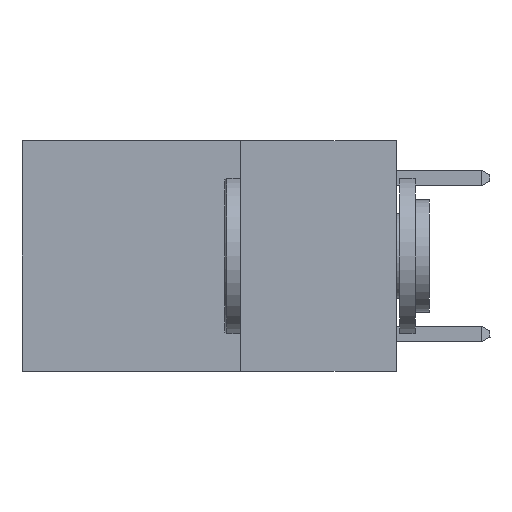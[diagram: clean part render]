
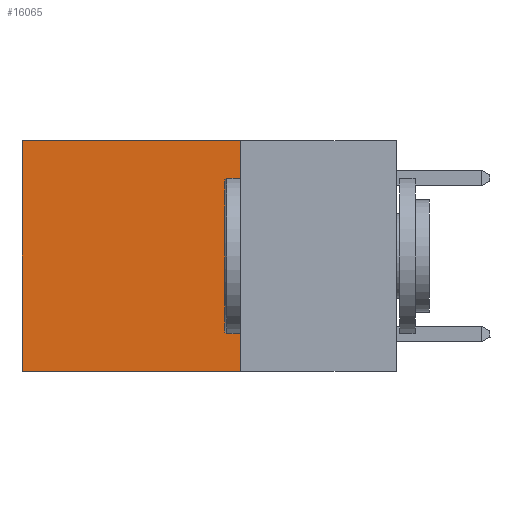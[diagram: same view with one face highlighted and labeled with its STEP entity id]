
A CAD part, left-side view. The second image highlights one B-rep face of the part: STEP entity #16065.
In plain terms, the highlighted planar face has unit normal (-1, 0, 0).
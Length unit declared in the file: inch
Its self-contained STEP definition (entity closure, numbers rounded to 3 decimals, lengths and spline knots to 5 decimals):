
#201 = VERTEX_POINT ( 'NONE', #2603 ) ;
#833 = VECTOR ( 'NONE', #1078, 39.37008 ) ;
#1078 = DIRECTION ( 'NONE',  ( 0., 1., 0. ) ) ;
#1350 = DIRECTION ( 'NONE',  ( 0., 0., -1. ) ) ;
#2198 = CARTESIAN_POINT ( 'NONE',  ( 0.2625, 0.25, 0. ) ) ;
#2397 = LINE ( 'NONE', #16668, #16218 ) ;
#2441 = FACE_OUTER_BOUND ( 'NONE', #7297, .T. ) ;
#2603 = CARTESIAN_POINT ( 'NONE',  ( 0.2625, 0.6, 0. ) ) ;
#3335 = ORIENTED_EDGE ( 'NONE', *, *, #18366, .T. ) ;
#4083 = EDGE_CURVE ( 'NONE', #201, #9149, #12155, .T. ) ;
#5642 = CARTESIAN_POINT ( 'NONE',  ( 0.2625, 0.25, 0. ) ) ;
#6493 = VECTOR ( 'NONE', #1350, 39.37008 ) ;
#7297 = EDGE_LOOP ( 'NONE', ( #19513, #7813, #15639, #3335 ) ) ;
#7525 = CARTESIAN_POINT ( 'NONE',  ( 0.2625, 0.25, -0.37 ) ) ;
#7813 = ORIENTED_EDGE ( 'NONE', *, *, #8856, .F. ) ;
#8118 = VERTEX_POINT ( 'NONE', #7525 ) ;
#8508 = DIRECTION ( 'NONE',  ( 1., 0., 0. ) ) ;
#8566 = DIRECTION ( 'NONE',  ( 0., 0., -1. ) ) ;
#8856 = EDGE_CURVE ( 'NONE', #8118, #9149, #19380, .T. ) ;
#9149 = VERTEX_POINT ( 'NONE', #13973 ) ;
#10589 = DIRECTION ( 'NONE',  ( 0., 0., -1. ) ) ;
#11029 = VERTEX_POINT ( 'NONE', #5642 ) ;
#11312 = CARTESIAN_POINT ( 'NONE',  ( 0.2625, 0.25, -0.37 ) ) ;
#12155 = LINE ( 'NONE', #16631, #6493 ) ;
#13565 = CARTESIAN_POINT ( 'NONE',  ( 0.2625, 0.25, 0. ) ) ;
#13973 = CARTESIAN_POINT ( 'NONE',  ( 0.2625, 0.6, -0.37 ) ) ;
#14780 = PLANE ( 'NONE',  #16892 ) ;
#15639 = ORIENTED_EDGE ( 'NONE', *, *, #18298, .F. ) ;
#15897 = DIRECTION ( 'NONE',  ( 0., 1., 0. ) ) ;
#16065 = ADVANCED_FACE ( 'NONE', ( #2441 ), #14780, .F. ) ;
#16218 = VECTOR ( 'NONE', #8566, 39.37008 ) ;
#16631 = CARTESIAN_POINT ( 'NONE',  ( 0.2625, 0.6, 0. ) ) ;
#16668 = CARTESIAN_POINT ( 'NONE',  ( 0.2625, 0.25, 0. ) ) ;
#16892 = AXIS2_PLACEMENT_3D ( 'NONE', #13565, #8508, #10589 ) ;
#18002 = LINE ( 'NONE', #2198, #833 ) ;
#18298 = EDGE_CURVE ( 'NONE', #11029, #8118, #2397, .T. ) ;
#18366 = EDGE_CURVE ( 'NONE', #11029, #201, #18002, .T. ) ;
#19059 = VECTOR ( 'NONE', #15897, 39.37008 ) ;
#19380 = LINE ( 'NONE', #11312, #19059 ) ;
#19513 = ORIENTED_EDGE ( 'NONE', *, *, #4083, .T. ) ;
